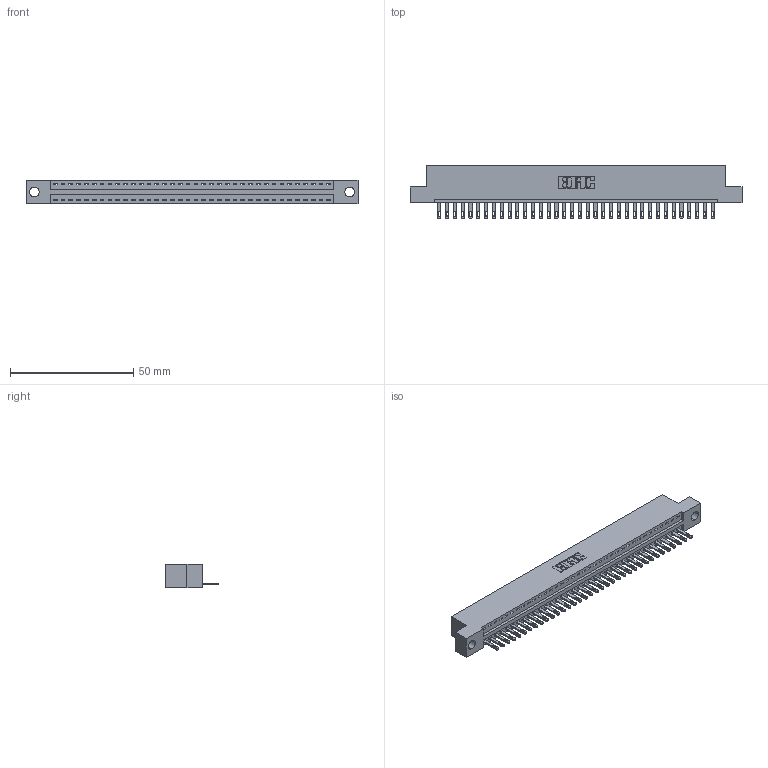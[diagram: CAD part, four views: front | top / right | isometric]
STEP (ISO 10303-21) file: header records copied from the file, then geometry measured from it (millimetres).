
FILE_DESCRIPTION (( 'STEP AP203' ), '1' );
FILE_NAME ('896-036-500-104.STEP', '2021-07-27T20:06:25', ( '' ), ( '' ), 'SwSTEP 2.0', 'SolidWorks 2020', '' );
FILE_SCHEMA (( 'CONFIG_CONTROL_DESIGN' ));
Length unit declared in the file: inch
Products named in the file (3): 896-036-500-104; 345-292-001_345-293-100; 846 Part_Flush Mounting Lugs - 0.156 Dia-TH
Assembly tree (37 placements, depth 2):
  896-036-500-104
    846 Part_Flush Mounting Lugs - 0.156 Dia-TH
    345-292-001_345-293-100  x36
Bounding box: 134.87 x 21.84 x 9.4 mm (x, y, z)
Volume: 12803.5 mm3; surface area: 15826.8 mm2
Topology: 37 solids, 37 shells, 2066 faces, 6377 edges, 4250 vertices
Faces by surface type: plane 1300, cylinder 766
Entity records: 23083 total; most frequent: CARTESIAN_POINT 3964, ORIENTED_EDGE 3934, DIRECTION 3507, EDGE_CURVE 1967, VECTOR 1687, LINE 1687, VERTEX_POINT 1310, AXIS2_PLACEMENT_3D 910
